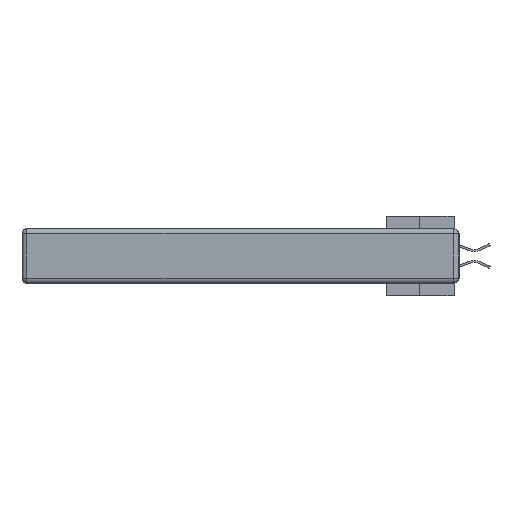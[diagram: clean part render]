
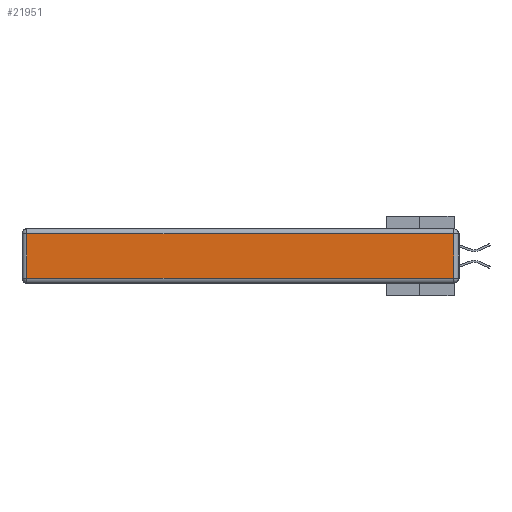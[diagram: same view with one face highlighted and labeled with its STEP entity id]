
A CAD part, left-side view. The second image highlights one B-rep face of the part: STEP entity #21951.
In plain terms, the highlighted planar face has unit normal (-1, 0, 0).
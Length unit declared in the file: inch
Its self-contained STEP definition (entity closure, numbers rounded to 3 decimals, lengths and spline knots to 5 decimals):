
#437 = VECTOR ( 'NONE', #40604, 39.37008 ) ;
#810 = VERTEX_POINT ( 'NONE', #11442 ) ;
#4441 = LINE ( 'NONE', #9104, #39883 ) ;
#5360 = LINE ( 'NONE', #18456, #437 ) ;
#6139 = ORIENTED_EDGE ( 'NONE', *, *, #29846, .T. ) ;
#7573 = CARTESIAN_POINT ( 'NONE',  ( 0., 2.75, -0.03 ) ) ;
#8264 = CARTESIAN_POINT ( 'NONE',  ( 0., 0.03, -0.313 ) ) ;
#9082 = EDGE_CURVE ( 'NONE', #11136, #39758, #39417, .T. ) ;
#9104 = CARTESIAN_POINT ( 'NONE',  ( 0., 0., -0.313 ) ) ;
#9112 = CARTESIAN_POINT ( 'NONE',  ( 0., 2.72, -0.313 ) ) ;
#10667 = FACE_OUTER_BOUND ( 'NONE', #23018, .T. ) ;
#11136 = VERTEX_POINT ( 'NONE', #8264 ) ;
#11442 = CARTESIAN_POINT ( 'NONE',  ( 0., 2.72, -0.03 ) ) ;
#13767 = ORIENTED_EDGE ( 'NONE', *, *, #28623, .T. ) ;
#14187 = DIRECTION ( 'NONE',  ( 0., 0., 1. ) ) ;
#16292 = VECTOR ( 'NONE', #14187, 39.37008 ) ;
#17409 = CARTESIAN_POINT ( 'NONE',  ( 0., 0.03, -0.03 ) ) ;
#18456 = CARTESIAN_POINT ( 'NONE',  ( 0., 2.72, -0.343 ) ) ;
#21150 = DIRECTION ( 'NONE',  ( 0., 0., 1. ) ) ;
#21762 = DIRECTION ( 'NONE',  ( 0., -1., 0. ) ) ;
#21951 = ADVANCED_FACE ( 'NONE', ( #10667 ), #36435, .T. ) ;
#23018 = EDGE_LOOP ( 'NONE', ( #6139, #25457, #40235, #13767 ) ) ;
#25457 = ORIENTED_EDGE ( 'NONE', *, *, #9082, .T. ) ;
#25831 = EDGE_CURVE ( 'NONE', #39758, #810, #28249, .T. ) ;
#28249 = LINE ( 'NONE', #7573, #30685 ) ;
#28604 = VERTEX_POINT ( 'NONE', #9112 ) ;
#28623 = EDGE_CURVE ( 'NONE', #810, #28604, #5360, .T. ) ;
#29078 = AXIS2_PLACEMENT_3D ( 'NONE', #36834, #33395, #21150 ) ;
#29846 = EDGE_CURVE ( 'NONE', #28604, #11136, #4441, .T. ) ;
#30685 = VECTOR ( 'NONE', #35520, 39.37008 ) ;
#33014 = CARTESIAN_POINT ( 'NONE',  ( 0., 0.03, -0.343 ) ) ;
#33395 = DIRECTION ( 'NONE',  ( -1., 0., 0. ) ) ;
#35520 = DIRECTION ( 'NONE',  ( 0., 1., 0. ) ) ;
#36435 = PLANE ( 'NONE',  #29078 ) ;
#36834 = CARTESIAN_POINT ( 'NONE',  ( 0., 0., -0.343 ) ) ;
#39417 = LINE ( 'NONE', #33014, #16292 ) ;
#39758 = VERTEX_POINT ( 'NONE', #17409 ) ;
#39883 = VECTOR ( 'NONE', #21762, 39.37008 ) ;
#40235 = ORIENTED_EDGE ( 'NONE', *, *, #25831, .T. ) ;
#40604 = DIRECTION ( 'NONE',  ( 0., 0., -1. ) ) ;
